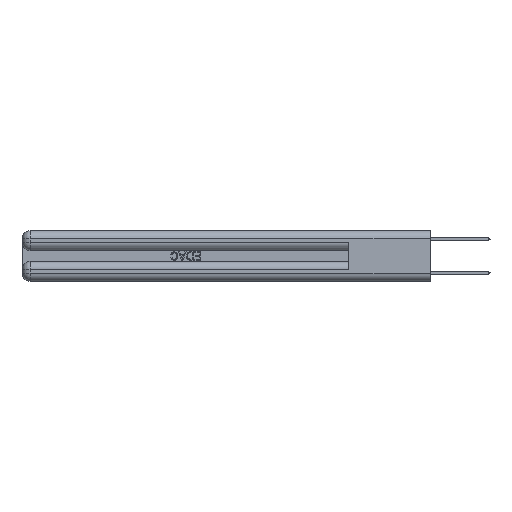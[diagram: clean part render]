
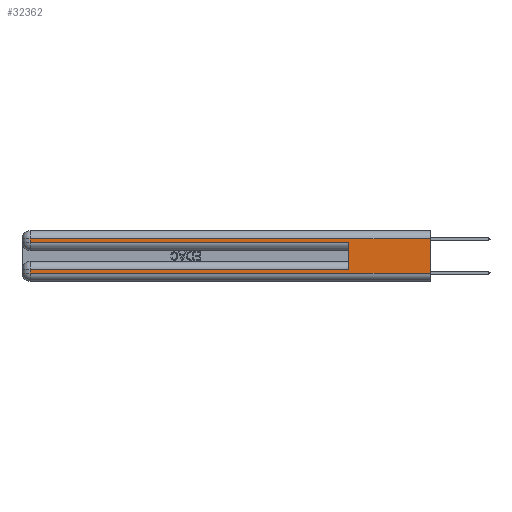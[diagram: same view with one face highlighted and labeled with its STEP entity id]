
A CAD part, left-side view. The second image highlights one B-rep face of the part: STEP entity #32362.
In plain terms, the highlighted planar face has unit normal (-1, 0, 0).
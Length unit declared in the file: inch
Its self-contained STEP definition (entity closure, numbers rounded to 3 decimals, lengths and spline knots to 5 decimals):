
#2798 = CARTESIAN_POINT ( 'NONE',  ( 0., 2.94, 0.37 ) ) ;
#3088 = CARTESIAN_POINT ( 'NONE',  ( 0., 0., 0.285 ) ) ;
#3104 = VERTEX_POINT ( 'NONE', #16923 ) ;
#3116 = LINE ( 'NONE', #32464, #25162 ) ;
#3220 = VERTEX_POINT ( 'NONE', #31075 ) ;
#5929 = EDGE_CURVE ( 'NONE', #27062, #9557, #17442, .T. ) ;
#5937 = ORIENTED_EDGE ( 'NONE', *, *, #20355, .T. ) ;
#6049 = EDGE_CURVE ( 'NONE', #31480, #3220, #30736, .T. ) ;
#8373 = CARTESIAN_POINT ( 'NONE',  ( 0., 0.6, 0.285 ) ) ;
#9121 = VECTOR ( 'NONE', #26789, 39.37008 ) ;
#9557 = VERTEX_POINT ( 'NONE', #29105 ) ;
#10030 = EDGE_CURVE ( 'NONE', #3104, #28614, #3116, .T. ) ;
#11754 = CARTESIAN_POINT ( 'NONE',  ( 0., 0., 0.06 ) ) ;
#12332 = CARTESIAN_POINT ( 'NONE',  ( 0., 2.94, 0.285 ) ) ;
#12908 = FACE_OUTER_BOUND ( 'NONE', #32740, .T. ) ;
#13650 = LINE ( 'NONE', #19007, #23854 ) ;
#13708 = VERTEX_POINT ( 'NONE', #12332 ) ;
#14777 = CARTESIAN_POINT ( 'NONE',  ( 0., 0., 0.31 ) ) ;
#14875 = DIRECTION ( 'NONE',  ( 0., 0., -1. ) ) ;
#15504 = ORIENTED_EDGE ( 'NONE', *, *, #6049, .T. ) ;
#15710 = ORIENTED_EDGE ( 'NONE', *, *, #5929, .T. ) ;
#16103 = VERTEX_POINT ( 'NONE', #23494 ) ;
#16246 = DIRECTION ( 'NONE',  ( 0., 1., 0. ) ) ;
#16714 = DIRECTION ( 'NONE',  ( 0., -1., 0. ) ) ;
#16923 = CARTESIAN_POINT ( 'NONE',  ( 0., 0.6, 0.085 ) ) ;
#16928 = DIRECTION ( 'NONE',  ( 0., -1., 0. ) ) ;
#17185 = EDGE_CURVE ( 'NONE', #3220, #13708, #28509, .T. ) ;
#17442 = LINE ( 'NONE', #11754, #17935 ) ;
#17616 = DIRECTION ( 'NONE',  ( 0., 1., 0. ) ) ;
#17935 = VECTOR ( 'NONE', #16928, 39.37008 ) ;
#18310 = CARTESIAN_POINT ( 'NONE',  ( 0., 0., 0.31 ) ) ;
#18652 = EDGE_CURVE ( 'NONE', #3104, #16103, #13650, .T. ) ;
#18728 = ORIENTED_EDGE ( 'NONE', *, *, #18652, .T. ) ;
#18808 = VECTOR ( 'NONE', #14875, 39.37008 ) ;
#19007 = CARTESIAN_POINT ( 'NONE',  ( 0., 0., 0.085 ) ) ;
#19098 = CARTESIAN_POINT ( 'NONE',  ( 0., 2.94, 0.06 ) ) ;
#20232 = CARTESIAN_POINT ( 'NONE',  ( 0., 2.94, 0.37 ) ) ;
#20355 = EDGE_CURVE ( 'NONE', #13708, #28614, #31923, .T. ) ;
#20699 = VECTOR ( 'NONE', #17616, 39.37008 ) ;
#20858 = ORIENTED_EDGE ( 'NONE', *, *, #10030, .F. ) ;
#21009 = AXIS2_PLACEMENT_3D ( 'NONE', #31218, #28805, #31575 ) ;
#21047 = LINE ( 'NONE', #23108, #24523 ) ;
#21099 = LINE ( 'NONE', #2798, #9121 ) ;
#23108 = CARTESIAN_POINT ( 'NONE',  ( 0., 0., 0.37 ) ) ;
#23146 = EDGE_CURVE ( 'NONE', #31480, #9557, #21047, .T. ) ;
#23361 = ORIENTED_EDGE ( 'NONE', *, *, #26052, .T. ) ;
#23494 = CARTESIAN_POINT ( 'NONE',  ( 0., 2.94, 0.085 ) ) ;
#23854 = VECTOR ( 'NONE', #16246, 39.37008 ) ;
#24523 = VECTOR ( 'NONE', #33965, 39.37008 ) ;
#25162 = VECTOR ( 'NONE', #27130, 39.37008 ) ;
#25532 = PLANE ( 'NONE',  #21009 ) ;
#26052 = EDGE_CURVE ( 'NONE', #16103, #27062, #21099, .T. ) ;
#26668 = VECTOR ( 'NONE', #16714, 39.37008 ) ;
#26789 = DIRECTION ( 'NONE',  ( 0., 0., -1. ) ) ;
#27062 = VERTEX_POINT ( 'NONE', #19098 ) ;
#27130 = DIRECTION ( 'NONE',  ( 0., 0., 1. ) ) ;
#28509 = LINE ( 'NONE', #20232, #18808 ) ;
#28614 = VERTEX_POINT ( 'NONE', #8373 ) ;
#28805 = DIRECTION ( 'NONE',  ( 1., 0., 0. ) ) ;
#29105 = CARTESIAN_POINT ( 'NONE',  ( 0., 0., 0.06 ) ) ;
#30736 = LINE ( 'NONE', #18310, #20699 ) ;
#30794 = ORIENTED_EDGE ( 'NONE', *, *, #23146, .F. ) ;
#30869 = ORIENTED_EDGE ( 'NONE', *, *, #17185, .T. ) ;
#31075 = CARTESIAN_POINT ( 'NONE',  ( 0., 2.94, 0.31 ) ) ;
#31218 = CARTESIAN_POINT ( 'NONE',  ( 0., 0., 0.37 ) ) ;
#31480 = VERTEX_POINT ( 'NONE', #14777 ) ;
#31575 = DIRECTION ( 'NONE',  ( 0., 0., -1. ) ) ;
#31923 = LINE ( 'NONE', #3088, #26668 ) ;
#32362 = ADVANCED_FACE ( 'NONE', ( #12908 ), #25532, .F. ) ;
#32464 = CARTESIAN_POINT ( 'NONE',  ( 0., 0.6, 0.145 ) ) ;
#32740 = EDGE_LOOP ( 'NONE', ( #30794, #15504, #30869, #5937, #20858, #18728, #23361, #15710 ) ) ;
#33965 = DIRECTION ( 'NONE',  ( 0., 0., -1. ) ) ;
